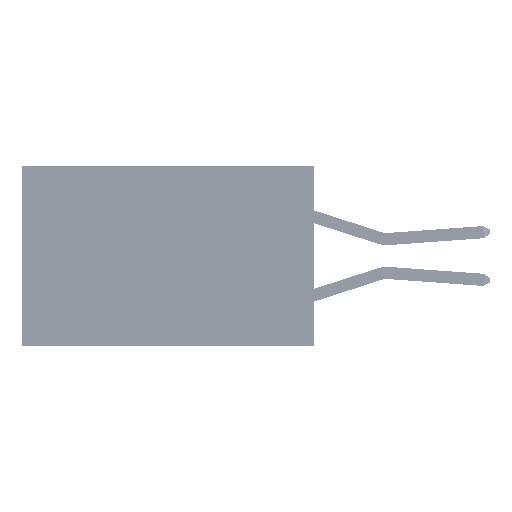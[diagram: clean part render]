
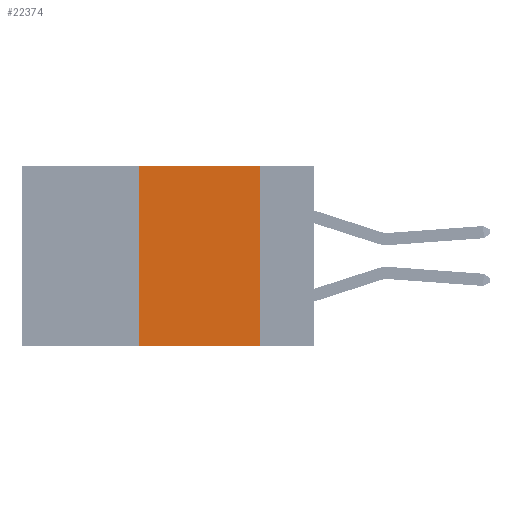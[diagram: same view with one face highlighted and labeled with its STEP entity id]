
A CAD part, left-side view. The second image highlights one B-rep face of the part: STEP entity #22374.
In plain terms, the highlighted planar face has unit normal (-1, 0, 0).
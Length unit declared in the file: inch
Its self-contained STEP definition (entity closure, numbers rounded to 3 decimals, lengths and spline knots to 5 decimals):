
#138 = CARTESIAN_POINT ( 'NONE',  ( 0., 0.36, 0. ) ) ;
#549 = ORIENTED_EDGE ( 'NONE', *, *, #33887, .F. ) ;
#1239 = LINE ( 'NONE', #18918, #30876 ) ;
#1769 = DIRECTION ( 'NONE',  ( 0., -1., 0. ) ) ;
#2313 = DIRECTION ( 'NONE',  ( 1., 0., 0. ) ) ;
#2314 = AXIS2_PLACEMENT_3D ( 'NONE', #17854, #2313, #48677 ) ;
#3325 = CARTESIAN_POINT ( 'NONE',  ( 0., 0.36, -0.37 ) ) ;
#3562 = DIRECTION ( 'NONE',  ( 0., 0., 1. ) ) ;
#9798 = DIRECTION ( 'NONE',  ( 0., -1., 0. ) ) ;
#12892 = EDGE_CURVE ( 'NONE', #33732, #27326, #1239, .T. ) ;
#14215 = LINE ( 'NONE', #40800, #36454 ) ;
#15378 = VECTOR ( 'NONE', #39707, 39.37008 ) ;
#16632 = VERTEX_POINT ( 'NONE', #19072 ) ;
#17183 = PLANE ( 'NONE',  #2314 ) ;
#17854 = CARTESIAN_POINT ( 'NONE',  ( 0., 0.6, 0. ) ) ;
#18918 = CARTESIAN_POINT ( 'NONE',  ( 0., 0.36, 0. ) ) ;
#19072 = CARTESIAN_POINT ( 'NONE',  ( 0., 0.11, -0.37 ) ) ;
#19447 = EDGE_CURVE ( 'NONE', #33732, #16632, #14215, .T. ) ;
#22002 = CARTESIAN_POINT ( 'NONE',  ( 0., 0.11, 0. ) ) ;
#22374 = ADVANCED_FACE ( 'NONE', ( #25265 ), #17183, .F. ) ;
#23595 = VERTEX_POINT ( 'NONE', #22002 ) ;
#24725 = ORIENTED_EDGE ( 'NONE', *, *, #29629, .F. ) ;
#25265 = FACE_OUTER_BOUND ( 'NONE', #34170, .T. ) ;
#27326 = VERTEX_POINT ( 'NONE', #138 ) ;
#29629 = EDGE_CURVE ( 'NONE', #27326, #23595, #49017, .T. ) ;
#30876 = VECTOR ( 'NONE', #3562, 39.37008 ) ;
#33732 = VERTEX_POINT ( 'NONE', #3325 ) ;
#33887 = EDGE_CURVE ( 'NONE', #23595, #16632, #38901, .T. ) ;
#34170 = EDGE_LOOP ( 'NONE', ( #549, #24725, #47994, #44375 ) ) ;
#36454 = VECTOR ( 'NONE', #9798, 39.37008 ) ;
#38901 = LINE ( 'NONE', #47619, #15378 ) ;
#39707 = DIRECTION ( 'NONE',  ( 0., 0., -1. ) ) ;
#40800 = CARTESIAN_POINT ( 'NONE',  ( 0., 0.6, -0.37 ) ) ;
#44375 = ORIENTED_EDGE ( 'NONE', *, *, #19447, .T. ) ;
#44484 = CARTESIAN_POINT ( 'NONE',  ( 0., 0.6, 0. ) ) ;
#46030 = VECTOR ( 'NONE', #1769, 39.37008 ) ;
#47619 = CARTESIAN_POINT ( 'NONE',  ( 0., 0.11, 0. ) ) ;
#47994 = ORIENTED_EDGE ( 'NONE', *, *, #12892, .F. ) ;
#48677 = DIRECTION ( 'NONE',  ( 0., 0., -1. ) ) ;
#49017 = LINE ( 'NONE', #44484, #46030 ) ;
